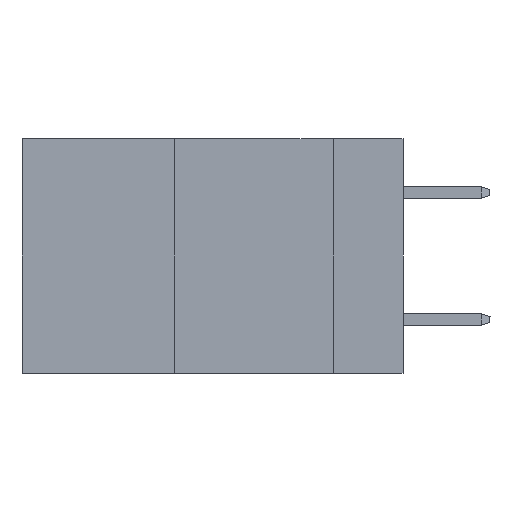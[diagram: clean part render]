
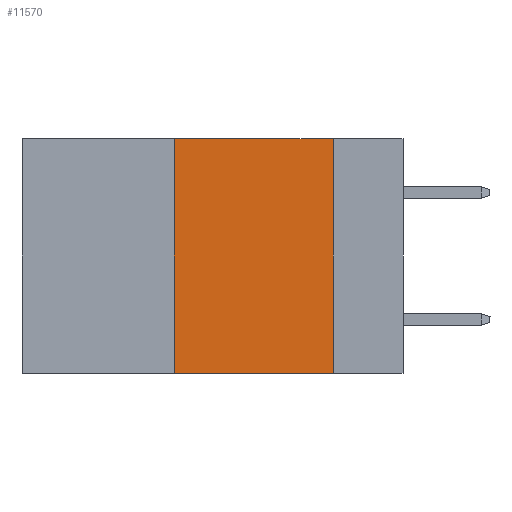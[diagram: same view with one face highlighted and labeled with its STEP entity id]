
A CAD part, left-side view. The second image highlights one B-rep face of the part: STEP entity #11570.
In plain terms, the highlighted planar face has unit normal (-1, 0, 0).
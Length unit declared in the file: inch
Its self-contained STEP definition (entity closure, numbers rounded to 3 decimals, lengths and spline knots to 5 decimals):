
#224 = PLANE ( 'NONE',  #6814 ) ;
#426 = CARTESIAN_POINT ( 'NONE',  ( 0., 0.6, 0. ) ) ;
#558 = CARTESIAN_POINT ( 'NONE',  ( 0., 0.6, -0.37 ) ) ;
#637 = CARTESIAN_POINT ( 'NONE',  ( 0., 0.36, -0.37 ) ) ;
#680 = VERTEX_POINT ( 'NONE', #1427 ) ;
#879 = VECTOR ( 'NONE', #6773, 39.37008 ) ;
#1238 = CARTESIAN_POINT ( 'NONE',  ( 0., 0.11, 0. ) ) ;
#1427 = CARTESIAN_POINT ( 'NONE',  ( 0., 0.11, -0.37 ) ) ;
#1519 = EDGE_CURVE ( 'NONE', #18716, #680, #16003, .T. ) ;
#2470 = ORIENTED_EDGE ( 'NONE', *, *, #6342, .F. ) ;
#2535 = CARTESIAN_POINT ( 'NONE',  ( 0., 0.11, 0. ) ) ;
#2612 = VERTEX_POINT ( 'NONE', #1238 ) ;
#5229 = LINE ( 'NONE', #6564, #15281 ) ;
#5951 = DIRECTION ( 'NONE',  ( 0., 0., 1. ) ) ;
#6293 = ORIENTED_EDGE ( 'NONE', *, *, #11310, .F. ) ;
#6342 = EDGE_CURVE ( 'NONE', #18716, #16744, #13379, .T. ) ;
#6564 = CARTESIAN_POINT ( 'NONE',  ( 0., 0.6, 0. ) ) ;
#6773 = DIRECTION ( 'NONE',  ( 0., -1., 0. ) ) ;
#6814 = AXIS2_PLACEMENT_3D ( 'NONE', #426, #12725, #8166 ) ;
#7969 = FACE_OUTER_BOUND ( 'NONE', #14835, .T. ) ;
#8166 = DIRECTION ( 'NONE',  ( 0., 0., -1. ) ) ;
#9251 = CARTESIAN_POINT ( 'NONE',  ( 0., 0.36, 0. ) ) ;
#10244 = VECTOR ( 'NONE', #5951, 39.37008 ) ;
#11310 = EDGE_CURVE ( 'NONE', #16744, #2612, #5229, .T. ) ;
#11570 = ADVANCED_FACE ( 'NONE', ( #7969 ), #224, .F. ) ;
#12725 = DIRECTION ( 'NONE',  ( 1., 0., 0. ) ) ;
#12747 = DIRECTION ( 'NONE',  ( 0., -1., 0. ) ) ;
#13379 = LINE ( 'NONE', #15105, #10244 ) ;
#13439 = DIRECTION ( 'NONE',  ( 0., 0., -1. ) ) ;
#14835 = EDGE_LOOP ( 'NONE', ( #15938, #6293, #2470, #19827 ) ) ;
#14964 = LINE ( 'NONE', #2535, #15689 ) ;
#15105 = CARTESIAN_POINT ( 'NONE',  ( 0., 0.36, 0. ) ) ;
#15281 = VECTOR ( 'NONE', #12747, 39.37008 ) ;
#15542 = EDGE_CURVE ( 'NONE', #2612, #680, #14964, .T. ) ;
#15689 = VECTOR ( 'NONE', #13439, 39.37008 ) ;
#15938 = ORIENTED_EDGE ( 'NONE', *, *, #15542, .F. ) ;
#16003 = LINE ( 'NONE', #558, #879 ) ;
#16744 = VERTEX_POINT ( 'NONE', #9251 ) ;
#18716 = VERTEX_POINT ( 'NONE', #637 ) ;
#19827 = ORIENTED_EDGE ( 'NONE', *, *, #1519, .T. ) ;
